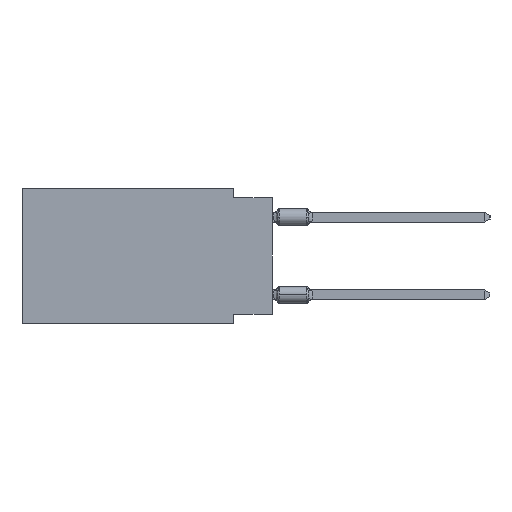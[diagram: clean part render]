
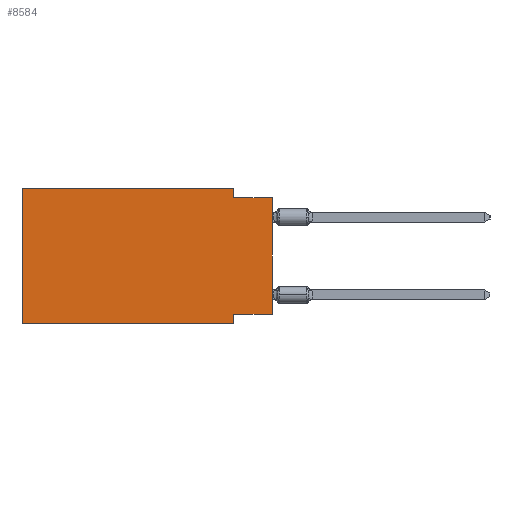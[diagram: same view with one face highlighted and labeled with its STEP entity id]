
A CAD part, left-side view. The second image highlights one B-rep face of the part: STEP entity #8584.
In plain terms, the highlighted planar face has unit normal (-1, 0, 0).
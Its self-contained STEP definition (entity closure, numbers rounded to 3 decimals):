
#274 = DIRECTION ( 'NONE',  ( 0., 0., -1. ) ) ;
#768 = EDGE_CURVE ( 'NONE', #27325, #6590, #22644, .T. ) ;
#2806 = EDGE_CURVE ( 'NONE', #33499, #9217, #10890, .T. ) ;
#3050 = DIRECTION ( 'NONE',  ( 1., 0., 0. ) ) ;
#3611 = DIRECTION ( 'NONE',  ( 0., 0., -1. ) ) ;
#3903 = CARTESIAN_POINT ( 'NONE',  ( 0., 2.54, -8.89 ) ) ;
#4919 = VECTOR ( 'NONE', #24886, 1000. ) ;
#5552 = CARTESIAN_POINT ( 'NONE',  ( 0., 16.383, -8.89 ) ) ;
#6590 = VERTEX_POINT ( 'NONE', #33436 ) ;
#8522 = FACE_OUTER_BOUND ( 'NONE', #14164, .T. ) ;
#8584 = ADVANCED_FACE ( 'NONE', ( #8522 ), #14743, .F. ) ;
#8660 = CARTESIAN_POINT ( 'NONE',  ( 0., 2.54, -8.255 ) ) ;
#9217 = VERTEX_POINT ( 'NONE', #12232 ) ;
#9785 = CARTESIAN_POINT ( 'NONE',  ( 0., 0., -8.255 ) ) ;
#10157 = VECTOR ( 'NONE', #14710, 1000. ) ;
#10299 = EDGE_CURVE ( 'NONE', #34111, #19433, #31416, .T. ) ;
#10502 = CARTESIAN_POINT ( 'NONE',  ( 0., 16.383, 0. ) ) ;
#10890 = LINE ( 'NONE', #16183, #22957 ) ;
#11689 = VECTOR ( 'NONE', #3611, 1000. ) ;
#12094 = LINE ( 'NONE', #34582, #11689 ) ;
#12113 = AXIS2_PLACEMENT_3D ( 'NONE', #20394, #3050, #17379 ) ;
#12232 = CARTESIAN_POINT ( 'NONE',  ( 0., 0., -0.635 ) ) ;
#12924 = ORIENTED_EDGE ( 'NONE', *, *, #21286, .T. ) ;
#13908 = VECTOR ( 'NONE', #274, 1000. ) ;
#14164 = EDGE_LOOP ( 'NONE', ( #12924, #17300, #20438, #18891, #27187, #32174, #21655, #23825 ) ) ;
#14710 = DIRECTION ( 'NONE',  ( 0., -1., 0. ) ) ;
#14743 = PLANE ( 'NONE',  #12113 ) ;
#14853 = LINE ( 'NONE', #29917, #18724 ) ;
#15966 = VERTEX_POINT ( 'NONE', #9785 ) ;
#16132 = LINE ( 'NONE', #19702, #24787 ) ;
#16183 = CARTESIAN_POINT ( 'NONE',  ( 0., 0., -0.635 ) ) ;
#16415 = EDGE_CURVE ( 'NONE', #34111, #27325, #14853, .T. ) ;
#16514 = VECTOR ( 'NONE', #34434, 1000. ) ;
#16549 = LINE ( 'NONE', #18128, #4919 ) ;
#17300 = ORIENTED_EDGE ( 'NONE', *, *, #2806, .F. ) ;
#17379 = DIRECTION ( 'NONE',  ( 0., 0., -1. ) ) ;
#18128 = CARTESIAN_POINT ( 'NONE',  ( 0., 0., 0. ) ) ;
#18724 = VECTOR ( 'NONE', #26896, 1000. ) ;
#18891 = ORIENTED_EDGE ( 'NONE', *, *, #768, .F. ) ;
#19433 = VERTEX_POINT ( 'NONE', #3903 ) ;
#19702 = CARTESIAN_POINT ( 'NONE',  ( 0., 0., -8.255 ) ) ;
#20172 = CARTESIAN_POINT ( 'NONE',  ( 0., 16.383, 0. ) ) ;
#20394 = CARTESIAN_POINT ( 'NONE',  ( 0., 16.383, 0. ) ) ;
#20438 = ORIENTED_EDGE ( 'NONE', *, *, #36073, .F. ) ;
#20549 = EDGE_CURVE ( 'NONE', #15966, #24185, #16132, .T. ) ;
#20813 = EDGE_CURVE ( 'NONE', #24185, #19433, #23108, .T. ) ;
#21286 = EDGE_CURVE ( 'NONE', #15966, #9217, #16549, .T. ) ;
#21655 = ORIENTED_EDGE ( 'NONE', *, *, #20813, .F. ) ;
#22407 = DIRECTION ( 'NONE',  ( 0., -1., 0. ) ) ;
#22644 = LINE ( 'NONE', #20172, #10157 ) ;
#22957 = VECTOR ( 'NONE', #22407, 1000. ) ;
#23108 = LINE ( 'NONE', #35374, #13908 ) ;
#23825 = ORIENTED_EDGE ( 'NONE', *, *, #20549, .F. ) ;
#24185 = VERTEX_POINT ( 'NONE', #8660 ) ;
#24444 = CARTESIAN_POINT ( 'NONE',  ( 0., 16.383, -8.89 ) ) ;
#24787 = VECTOR ( 'NONE', #31052, 1000. ) ;
#24886 = DIRECTION ( 'NONE',  ( 0., 0., 1. ) ) ;
#26896 = DIRECTION ( 'NONE',  ( 0., 0., 1. ) ) ;
#27187 = ORIENTED_EDGE ( 'NONE', *, *, #16415, .F. ) ;
#27325 = VERTEX_POINT ( 'NONE', #10502 ) ;
#27330 = CARTESIAN_POINT ( 'NONE',  ( 0., 2.54, -0.635 ) ) ;
#29917 = CARTESIAN_POINT ( 'NONE',  ( 0., 16.383, 0. ) ) ;
#31052 = DIRECTION ( 'NONE',  ( 0., 1., 0. ) ) ;
#31416 = LINE ( 'NONE', #5552, #16514 ) ;
#32174 = ORIENTED_EDGE ( 'NONE', *, *, #10299, .T. ) ;
#33436 = CARTESIAN_POINT ( 'NONE',  ( 0., 2.54, 0. ) ) ;
#33499 = VERTEX_POINT ( 'NONE', #27330 ) ;
#34111 = VERTEX_POINT ( 'NONE', #24444 ) ;
#34434 = DIRECTION ( 'NONE',  ( 0., -1., 0. ) ) ;
#34582 = CARTESIAN_POINT ( 'NONE',  ( 0., 2.54, 0. ) ) ;
#35374 = CARTESIAN_POINT ( 'NONE',  ( 0., 2.54, -8.89 ) ) ;
#36073 = EDGE_CURVE ( 'NONE', #6590, #33499, #12094, .T. ) ;
